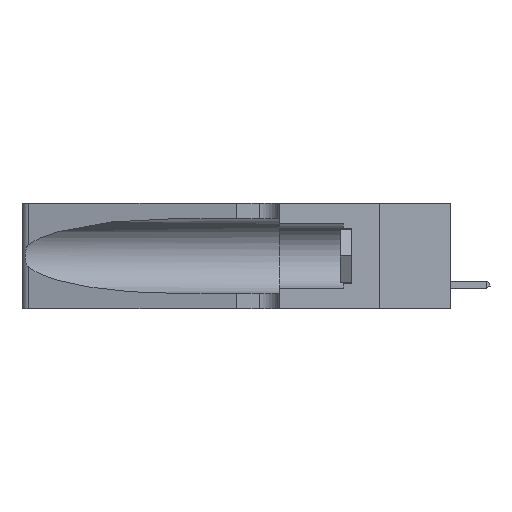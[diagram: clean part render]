
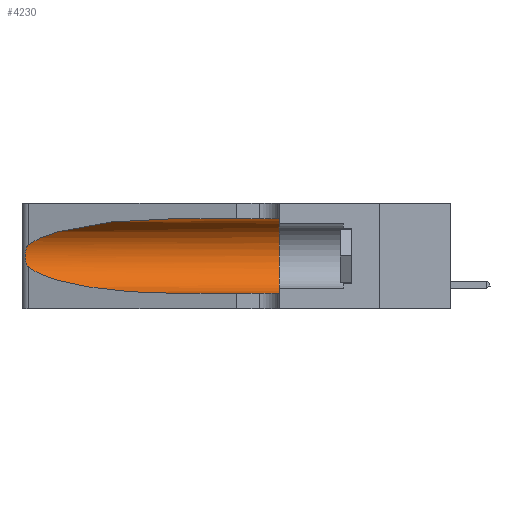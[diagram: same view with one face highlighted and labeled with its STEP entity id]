
A CAD part, left-side view. The second image highlights one B-rep face of the part: STEP entity #4230.
In plain terms, the highlighted cylindrical face has radius 3.308 mm (diameter 6.617 mm), a partial arc.
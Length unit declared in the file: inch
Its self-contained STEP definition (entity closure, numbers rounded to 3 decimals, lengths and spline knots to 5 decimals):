
#553 = CARTESIAN_POINT ( 'NONE',  ( 0.1305, 0.35, 0.05475 ) ) ;
#671 = EDGE_CURVE ( 'NONE', #9676, #13514, #1095, .T. ) ;
#712 = ORIENTED_EDGE ( 'NONE', *, *, #7615, .T. ) ;
#877 = EDGE_LOOP ( 'NONE', ( #9419, #6064, #712, #11177, #9430, #11007 ) ) ;
#1095 = B_SPLINE_CURVE_WITH_KNOTS ( 'NONE', 3,
 ( #13898, #1283, #3640, #3869, #13840, #15180, #6215, #15124, #7520, #5029, #2448, #12678, #6322, #13956 ),
 .UNSPECIFIED., .F., .F.,
 ( 4, 2, 2, 2, 2, 2, 4 ),
 ( 0., 0.00027, 0.00053, 0.00107, 0.0016, 0.00187, 0.00214 ),
 .UNSPECIFIED. ) ;
#1283 = CARTESIAN_POINT ( 'NONE',  ( 0.25555, 1.22994, 0.2215 ) ) ;
#1374 = CIRCLE ( 'NONE', #4259, 0.13025 ) ;
#1413 = CARTESIAN_POINT ( 'NONE',  ( 0.1305, 0.72297, 0.05475 ) ) ;
#2204 = CARTESIAN_POINT ( 'NONE',  ( 0.18966, 0.96281, 0.31525 ) ) ;
#2448 = CARTESIAN_POINT ( 'NONE',  ( 0.25789, 1.23486, 0.15765 ) ) ;
#2843 = CARTESIAN_POINT ( 'NONE',  ( 0.25487, 1.22718, 0.14631 ) ) ;
#3640 = CARTESIAN_POINT ( 'NONE',  ( 0.25639, 1.23184, 0.21858 ) ) ;
#3869 = CARTESIAN_POINT ( 'NONE',  ( 0.25787, 1.23484, 0.2124 ) ) ;
#4230 = ADVANCED_FACE ( 'NONE', ( #15072 ), #6492, .F. ) ;
#4259 = AXIS2_PLACEMENT_3D ( 'NONE', #14109, #14010, #11405 ) ;
#4516 = VERTEX_POINT ( 'NONE', #1413 ) ;
#4663 = DIRECTION ( 'NONE',  ( 0., -1., 0. ) ) ;
#5029 = CARTESIAN_POINT ( 'NONE',  ( 0.25856, 1.23593, 0.16098 ) ) ;
#5052 = VERTEX_POINT ( 'NONE', #553 ) ;
#5449 = LINE ( 'NONE', #5650, #16004 ) ;
#5650 = CARTESIAN_POINT ( 'NONE',  ( 0.1305, 1.61858, 0.05475 ) ) ;
#5757 = EDGE_CURVE ( 'NONE', #15748, #8338, #7616, .T. ) ;
#5800 =( BOUNDED_CURVE ( )  B_SPLINE_CURVE ( 3, ( #13866, #2204, #8753, #6122 ),
 .UNSPECIFIED., .F., .F. ) 
 B_SPLINE_CURVE_WITH_KNOTS ( ( 4, 4 ),
 ( 1.5708, 2.84003 ),
 .UNSPECIFIED. ) 
 CURVE ( )  GEOMETRIC_REPRESENTATION_ITEM ( )  RATIONAL_B_SPLINE_CURVE ( ( 1., 0.87, 0.87, 1. ) ) 
 REPRESENTATION_ITEM ( '' )  );
#6064 = ORIENTED_EDGE ( 'NONE', *, *, #671, .T. ) ;
#6122 = CARTESIAN_POINT ( 'NONE',  ( 0.25487, 1.22718, 0.22369 ) ) ;
#6215 = CARTESIAN_POINT ( 'NONE',  ( 0.26075, 1.23896, 0.19203 ) ) ;
#6322 = CARTESIAN_POINT ( 'NONE',  ( 0.25555, 1.22993, 0.14849 ) ) ;
#6492 = CYLINDRICAL_SURFACE ( 'NONE', #11498, 0.13025 ) ;
#6981 = DIRECTION ( 'NONE',  ( 0., 0., -1. ) ) ;
#7520 = CARTESIAN_POINT ( 'NONE',  ( 0.26017, 1.23833, 0.17102 ) ) ;
#7615 = EDGE_CURVE ( 'NONE', #13514, #4516, #10485, .T. ) ;
#7616 = LINE ( 'NONE', #12264, #12641 ) ;
#7802 = CARTESIAN_POINT ( 'NONE',  ( 0.25487, 1.22718, 0.22369 ) ) ;
#8338 = VERTEX_POINT ( 'NONE', #12621 ) ;
#8689 = EDGE_CURVE ( 'NONE', #15748, #9676, #5800, .T. ) ;
#8753 = CARTESIAN_POINT ( 'NONE',  ( 0.2373, 1.15595, 0.28018 ) ) ;
#9233 = CARTESIAN_POINT ( 'NONE',  ( 0.2373, 1.15595, 0.08982 ) ) ;
#9419 = ORIENTED_EDGE ( 'NONE', *, *, #8689, .T. ) ;
#9430 = ORIENTED_EDGE ( 'NONE', *, *, #16243, .F. ) ;
#9676 = VERTEX_POINT ( 'NONE', #7802 ) ;
#10004 = DIRECTION ( 'NONE',  ( 0., -1., 0. ) ) ;
#10485 =( BOUNDED_CURVE ( )  B_SPLINE_CURVE ( 3, ( #2843, #9233, #11451, #12795 ),
 .UNSPECIFIED., .F., .F. ) 
 B_SPLINE_CURVE_WITH_KNOTS ( ( 4, 4 ),
 ( 3.44316, 4.71239 ),
 .UNSPECIFIED. ) 
 CURVE ( )  GEOMETRIC_REPRESENTATION_ITEM ( )  RATIONAL_B_SPLINE_CURVE ( ( 1., 0.87, 0.87, 1. ) ) 
 REPRESENTATION_ITEM ( '' )  );
#10667 = DIRECTION ( 'NONE',  ( 0., -1., 0. ) ) ;
#10943 = EDGE_CURVE ( 'NONE', #4516, #5052, #5449, .T. ) ;
#11007 = ORIENTED_EDGE ( 'NONE', *, *, #5757, .F. ) ;
#11177 = ORIENTED_EDGE ( 'NONE', *, *, #10943, .T. ) ;
#11405 = DIRECTION ( 'NONE',  ( 0., 0., 1. ) ) ;
#11451 = CARTESIAN_POINT ( 'NONE',  ( 0.18966, 0.96281, 0.05475 ) ) ;
#11456 = CARTESIAN_POINT ( 'NONE',  ( 0.1305, 1.61858, 0.185 ) ) ;
#11498 = AXIS2_PLACEMENT_3D ( 'NONE', #11456, #10004, #6981 ) ;
#12263 = CARTESIAN_POINT ( 'NONE',  ( 0.1305, 0.72297, 0.31525 ) ) ;
#12264 = CARTESIAN_POINT ( 'NONE',  ( 0.1305, 1.61858, 0.31525 ) ) ;
#12621 = CARTESIAN_POINT ( 'NONE',  ( 0.1305, 0.35, 0.31525 ) ) ;
#12641 = VECTOR ( 'NONE', #4663, 39.37008 ) ;
#12678 = CARTESIAN_POINT ( 'NONE',  ( 0.25639, 1.23186, 0.15144 ) ) ;
#12795 = CARTESIAN_POINT ( 'NONE',  ( 0.1305, 0.72297, 0.05475 ) ) ;
#13514 = VERTEX_POINT ( 'NONE', #14246 ) ;
#13840 = CARTESIAN_POINT ( 'NONE',  ( 0.25854, 1.2359, 0.20912 ) ) ;
#13866 = CARTESIAN_POINT ( 'NONE',  ( 0.1305, 0.72297, 0.31525 ) ) ;
#13898 = CARTESIAN_POINT ( 'NONE',  ( 0.25487, 1.22718, 0.22369 ) ) ;
#13956 = CARTESIAN_POINT ( 'NONE',  ( 0.25487, 1.22718, 0.14631 ) ) ;
#14010 = DIRECTION ( 'NONE',  ( 0., 1., 0. ) ) ;
#14109 = CARTESIAN_POINT ( 'NONE',  ( 0.1305, 0.35, 0.185 ) ) ;
#14246 = CARTESIAN_POINT ( 'NONE',  ( 0.25487, 1.22718, 0.14631 ) ) ;
#15072 = FACE_OUTER_BOUND ( 'NONE', #877, .T. ) ;
#15124 = CARTESIAN_POINT ( 'NONE',  ( 0.26075, 1.23896, 0.178 ) ) ;
#15180 = CARTESIAN_POINT ( 'NONE',  ( 0.26018, 1.23835, 0.19895 ) ) ;
#15748 = VERTEX_POINT ( 'NONE', #12263 ) ;
#16004 = VECTOR ( 'NONE', #10667, 39.37008 ) ;
#16243 = EDGE_CURVE ( 'NONE', #8338, #5052, #1374, .T. ) ;
